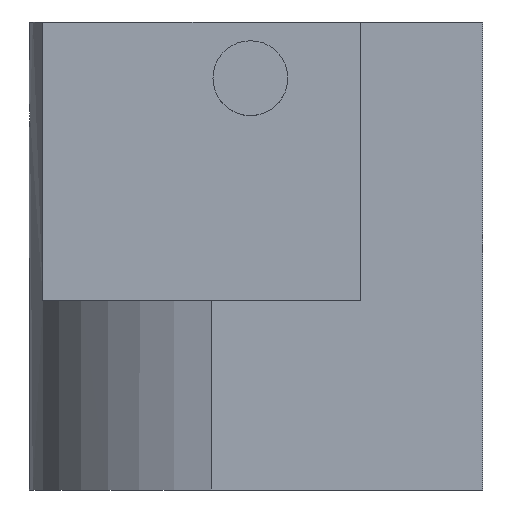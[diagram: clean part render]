
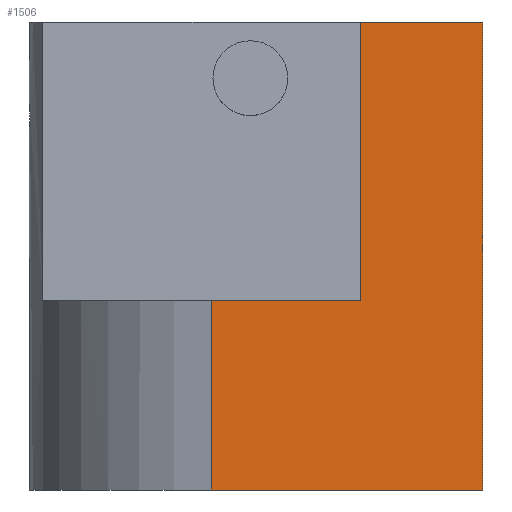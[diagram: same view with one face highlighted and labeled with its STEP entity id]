
A CAD part, left-side view. The second image highlights one B-rep face of the part: STEP entity #1506.
In plain terms, the highlighted planar face has unit normal (-1, 0, 0).
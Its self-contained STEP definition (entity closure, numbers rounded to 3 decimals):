
#92 = CARTESIAN_POINT ( 'NONE',  ( -58.909, 11.39, -139.424 ) ) ;
#102 = CARTESIAN_POINT ( 'NONE',  ( -58.909, -28.313, -65. ) ) ;
#105 = EDGE_CURVE ( 'NONE', #1642, #377, #672, .T. ) ;
#171 = LINE ( 'NONE', #312, #445 ) ;
#208 = EDGE_CURVE ( 'NONE', #1027, #1276, #593, .T. ) ;
#293 = VECTOR ( 'NONE', #1385, 1000. ) ;
#312 = CARTESIAN_POINT ( 'NONE',  ( -58.909, -28.313, -40. ) ) ;
#318 = LINE ( 'NONE', #1512, #1689 ) ;
#319 = VECTOR ( 'NONE', #1064, 1000. ) ;
#341 = ORIENTED_EDGE ( 'NONE', *, *, #1213, .F. ) ;
#377 = VERTEX_POINT ( 'NONE', #92 ) ;
#437 = CARTESIAN_POINT ( 'NONE',  ( -58.909, -61., -190. ) ) ;
#445 = VECTOR ( 'NONE', #590, 1000. ) ;
#518 = LINE ( 'NONE', #1035, #821 ) ;
#528 = DIRECTION ( 'NONE',  ( 0., -1., 0. ) ) ;
#580 = PLANE ( 'NONE',  #1202 ) ;
#590 = DIRECTION ( 'NONE',  ( 0., 0., 1. ) ) ;
#593 = LINE ( 'NONE', #1624, #293 ) ;
#616 = FACE_OUTER_BOUND ( 'NONE', #1688, .T. ) ;
#670 = CARTESIAN_POINT ( 'NONE',  ( -58.909, -61., -190. ) ) ;
#672 = LINE ( 'NONE', #1057, #319 ) ;
#728 = DIRECTION ( 'NONE',  ( 0., 1., 0. ) ) ;
#821 = VECTOR ( 'NONE', #528, 1000. ) ;
#840 = DIRECTION ( 'NONE',  ( 1., 0., 0. ) ) ;
#845 = VERTEX_POINT ( 'NONE', #1315 ) ;
#846 = CARTESIAN_POINT ( 'NONE',  ( -58.909, 11.39, -190. ) ) ;
#872 = ORIENTED_EDGE ( 'NONE', *, *, #208, .T. ) ;
#1027 = VERTEX_POINT ( 'NONE', #1499 ) ;
#1035 = CARTESIAN_POINT ( 'NONE',  ( -58.909, -28.313, -139.424 ) ) ;
#1057 = CARTESIAN_POINT ( 'NONE',  ( -58.909, 11.39, -190. ) ) ;
#1064 = DIRECTION ( 'NONE',  ( 0., 0., 1. ) ) ;
#1110 = VECTOR ( 'NONE', #1639, 1000. ) ;
#1155 = CARTESIAN_POINT ( 'NONE',  ( -58.909, 11.39, -190. ) ) ;
#1202 = AXIS2_PLACEMENT_3D ( 'NONE', #846, #840, #1519 ) ;
#1213 = EDGE_CURVE ( 'NONE', #377, #845, #518, .T. ) ;
#1276 = VERTEX_POINT ( 'NONE', #102 ) ;
#1315 = CARTESIAN_POINT ( 'NONE',  ( -58.909, -28.313, -139.424 ) ) ;
#1340 = VERTEX_POINT ( 'NONE', #437 ) ;
#1381 = ORIENTED_EDGE ( 'NONE', *, *, #1463, .F. ) ;
#1385 = DIRECTION ( 'NONE',  ( 0., 1., 0. ) ) ;
#1397 = EDGE_CURVE ( 'NONE', #1340, #1027, #1629, .T. ) ;
#1463 = EDGE_CURVE ( 'NONE', #1340, #1642, #318, .T. ) ;
#1494 = ORIENTED_EDGE ( 'NONE', *, *, #1397, .T. ) ;
#1499 = CARTESIAN_POINT ( 'NONE',  ( -58.909, -61., -65. ) ) ;
#1506 = ADVANCED_FACE ( 'NONE', ( #616 ), #580, .F. ) ;
#1512 = CARTESIAN_POINT ( 'NONE',  ( -58.909, 11.39, -190. ) ) ;
#1519 = DIRECTION ( 'NONE',  ( 0., 1., 0. ) ) ;
#1521 = EDGE_CURVE ( 'NONE', #845, #1276, #171, .T. ) ;
#1624 = CARTESIAN_POINT ( 'NONE',  ( -58.909, 11.39, -65. ) ) ;
#1629 = LINE ( 'NONE', #670, #1110 ) ;
#1638 = ORIENTED_EDGE ( 'NONE', *, *, #1521, .F. ) ;
#1639 = DIRECTION ( 'NONE',  ( 0., 0., 1. ) ) ;
#1642 = VERTEX_POINT ( 'NONE', #1155 ) ;
#1648 = ORIENTED_EDGE ( 'NONE', *, *, #105, .F. ) ;
#1688 = EDGE_LOOP ( 'NONE', ( #872, #1638, #341, #1648, #1381, #1494 ) ) ;
#1689 = VECTOR ( 'NONE', #728, 1000. ) ;
